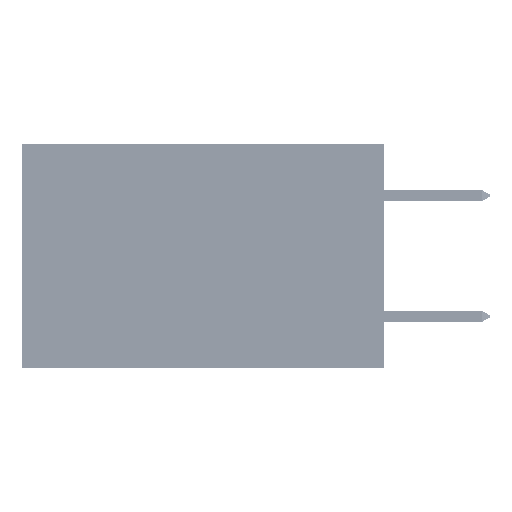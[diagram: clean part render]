
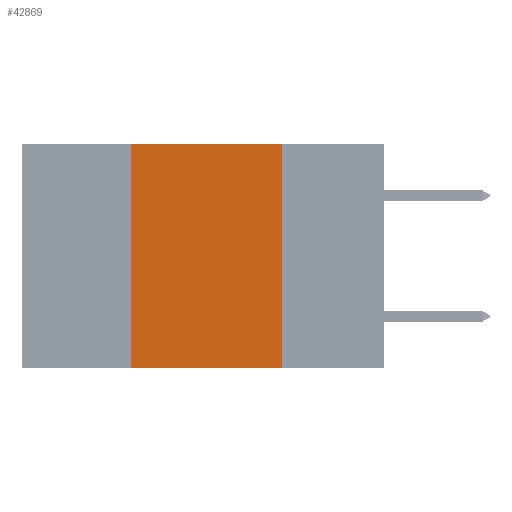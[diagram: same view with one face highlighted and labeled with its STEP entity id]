
A CAD part, left-side view. The second image highlights one B-rep face of the part: STEP entity #42869.
In plain terms, the highlighted planar face has unit normal (-1, 0, 0).
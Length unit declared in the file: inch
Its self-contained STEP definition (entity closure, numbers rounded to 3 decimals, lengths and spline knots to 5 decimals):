
#3028 = ORIENTED_EDGE ( 'NONE', *, *, #41988, .F. ) ;
#6298 = CARTESIAN_POINT ( 'NONE',  ( 0., 0.17, -0.37 ) ) ;
#6877 = FACE_OUTER_BOUND ( 'NONE', #13118, .T. ) ;
#8329 = LINE ( 'NONE', #20492, #37644 ) ;
#9695 = CARTESIAN_POINT ( 'NONE',  ( 0., 0.6, -0.37 ) ) ;
#11294 = VECTOR ( 'NONE', #26163, 39.37008 ) ;
#13118 = EDGE_LOOP ( 'NONE', ( #3028, #23961, #44748, #36949 ) ) ;
#15803 = LINE ( 'NONE', #44852, #25408 ) ;
#18237 = VERTEX_POINT ( 'NONE', #36278 ) ;
#18483 = CARTESIAN_POINT ( 'NONE',  ( 0., 0.6, 0. ) ) ;
#20492 = CARTESIAN_POINT ( 'NONE',  ( 0., 0.17, 0. ) ) ;
#20540 = LINE ( 'NONE', #36962, #34923 ) ;
#22434 = VERTEX_POINT ( 'NONE', #36665 ) ;
#22548 = VERTEX_POINT ( 'NONE', #6298 ) ;
#23961 = ORIENTED_EDGE ( 'NONE', *, *, #38345, .F. ) ;
#24269 = DIRECTION ( 'NONE',  ( 0., 0., -1. ) ) ;
#24425 = DIRECTION ( 'NONE',  ( 0., 0., 1. ) ) ;
#25408 = VECTOR ( 'NONE', #24425, 39.37008 ) ;
#26163 = DIRECTION ( 'NONE',  ( 0., -1., 0. ) ) ;
#28822 = CARTESIAN_POINT ( 'NONE',  ( 0., 0.42, 0. ) ) ;
#30221 = LINE ( 'NONE', #9695, #11294 ) ;
#34478 = VERTEX_POINT ( 'NONE', #28822 ) ;
#34910 = DIRECTION ( 'NONE',  ( 0., 0., -1. ) ) ;
#34923 = VECTOR ( 'NONE', #49053, 39.37008 ) ;
#36278 = CARTESIAN_POINT ( 'NONE',  ( 0., 0.17, 0. ) ) ;
#36665 = CARTESIAN_POINT ( 'NONE',  ( 0., 0.42, -0.37 ) ) ;
#36949 = ORIENTED_EDGE ( 'NONE', *, *, #50354, .T. ) ;
#36962 = CARTESIAN_POINT ( 'NONE',  ( 0., 0.6, 0. ) ) ;
#37290 = EDGE_CURVE ( 'NONE', #22434, #34478, #15803, .T. ) ;
#37644 = VECTOR ( 'NONE', #24269, 39.37008 ) ;
#38345 = EDGE_CURVE ( 'NONE', #34478, #18237, #20540, .T. ) ;
#39712 = DIRECTION ( 'NONE',  ( 1., 0., 0. ) ) ;
#40294 = AXIS2_PLACEMENT_3D ( 'NONE', #18483, #39712, #34910 ) ;
#41988 = EDGE_CURVE ( 'NONE', #18237, #22548, #8329, .T. ) ;
#42869 = ADVANCED_FACE ( 'NONE', ( #6877 ), #47018, .F. ) ;
#44748 = ORIENTED_EDGE ( 'NONE', *, *, #37290, .F. ) ;
#44852 = CARTESIAN_POINT ( 'NONE',  ( 0., 0.42, 0. ) ) ;
#47018 = PLANE ( 'NONE',  #40294 ) ;
#49053 = DIRECTION ( 'NONE',  ( 0., -1., 0. ) ) ;
#50354 = EDGE_CURVE ( 'NONE', #22434, #22548, #30221, .T. ) ;
